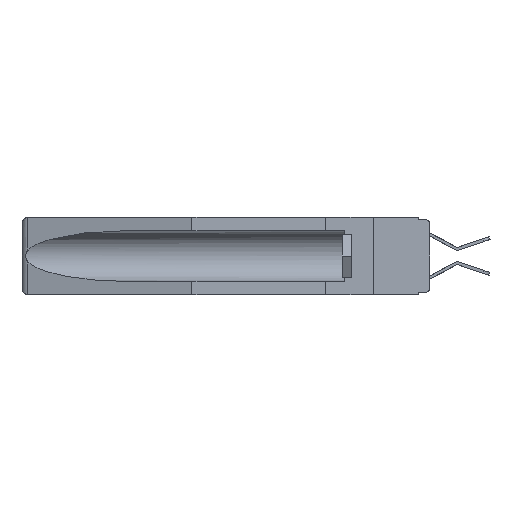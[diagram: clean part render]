
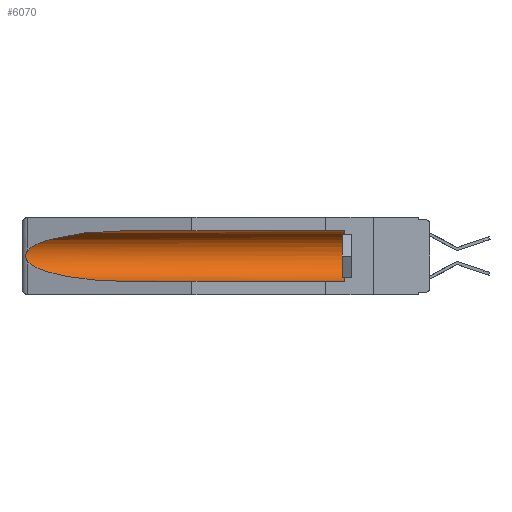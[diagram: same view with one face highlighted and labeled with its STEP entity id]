
A CAD part, left-side view. The second image highlights one B-rep face of the part: STEP entity #6070.
In plain terms, the highlighted cylindrical face has radius 2.857 mm (diameter 5.715 mm), a partial arc.
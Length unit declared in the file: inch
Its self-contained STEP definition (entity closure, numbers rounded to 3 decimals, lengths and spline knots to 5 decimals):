
#54 = EDGE_CURVE ( 'NONE', #11934, #7314, #14730, .T. ) ;
#150 = CARTESIAN_POINT ( 'NONE',  ( 0.21114, 1.30732, -0.059 ) ) ;
#220 =( BOUNDED_CURVE ( )  B_SPLINE_CURVE ( 3, ( #12397, #5140, #10967, #10677 ),
 .UNSPECIFIED., .F., .F. ) 
 B_SPLINE_CURVE_WITH_KNOTS ( ( 4, 4 ),
 ( 0.1948, 1.5708 ),
 .UNSPECIFIED. ) 
 CURVE ( )  GEOMETRIC_REPRESENTATION_ITEM ( )  RATIONAL_B_SPLINE_CURVE ( ( 1., 0.848, 0.848, 1. ) ) 
 REPRESENTATION_ITEM ( '' )  );
#445 = CARTESIAN_POINT ( 'NONE',  ( 0.2673, 1.5327, -0.16383 ) ) ;
#542 = ORIENTED_EDGE ( 'NONE', *, *, #2646, .T. ) ;
#723 = CARTESIAN_POINT ( 'NONE',  ( 0.2673, 1.53269, -0.17917 ) ) ;
#1757 = CARTESIAN_POINT ( 'NONE',  ( 0.155, 1.07973, -0.059 ) ) ;
#2565 = AXIS2_PLACEMENT_3D ( 'NONE', #5323, #18333, #18431 ) ;
#2646 = EDGE_CURVE ( 'NONE', #7314, #17627, #11357, .T. ) ;
#2702 = LINE ( 'NONE', #9964, #5491 ) ;
#3392 = DIRECTION ( 'NONE',  ( 0., 1., 0. ) ) ;
#3399 = CARTESIAN_POINT ( 'NONE',  ( 0.155, 0.126, -0.1715 ) ) ;
#4079 = AXIS2_PLACEMENT_3D ( 'NONE', #3399, #6447, #10950 ) ;
#4982 = ORIENTED_EDGE ( 'NONE', *, *, #9764, .T. ) ;
#5024 = CARTESIAN_POINT ( 'NONE',  ( 0.26597, 1.52961, -0.15275 ) ) ;
#5117 = CARTESIAN_POINT ( 'NONE',  ( 0.26537, 1.52718, -0.19328 ) ) ;
#5140 = CARTESIAN_POINT ( 'NONE',  ( 0.25451, 1.48313, -0.24835 ) ) ;
#5323 = CARTESIAN_POINT ( 'NONE',  ( 0.155, -0.30754, -0.1715 ) ) ;
#5491 = VECTOR ( 'NONE', #18487, 39.37008 ) ;
#6070 = ADVANCED_FACE ( 'NONE', ( #9517 ), #11938, .F. ) ;
#6447 = DIRECTION ( 'NONE',  ( 0., -1., 0. ) ) ;
#7170 = CARTESIAN_POINT ( 'NONE',  ( 0.155, 0.126, -0.284 ) ) ;
#7314 = VERTEX_POINT ( 'NONE', #8715 ) ;
#7609 = ORIENTED_EDGE ( 'NONE', *, *, #12559, .T. ) ;
#7975 = CARTESIAN_POINT ( 'NONE',  ( 0.26655, 1.53094, -0.18657 ) ) ;
#8081 = CARTESIAN_POINT ( 'NONE',  ( 0.2675, 1.53308, -0.17534 ) ) ;
#8715 = CARTESIAN_POINT ( 'NONE',  ( 0.26537, 1.52718, -0.14972 ) ) ;
#9391 = ORIENTED_EDGE ( 'NONE', *, *, #18700, .T. ) ;
#9517 = FACE_OUTER_BOUND ( 'NONE', #13673, .T. ) ;
#9764 = EDGE_CURVE ( 'NONE', #12864, #11934, #10479, .T. ) ;
#9964 = CARTESIAN_POINT ( 'NONE',  ( 0.155, -0.30754, -0.284 ) ) ;
#10094 = CARTESIAN_POINT ( 'NONE',  ( 0.25451, 1.48313, -0.09465 ) ) ;
#10386 = CARTESIAN_POINT ( 'NONE',  ( 0.155, 0.126, -0.059 ) ) ;
#10479 = LINE ( 'NONE', #15146, #15121 ) ;
#10677 = CARTESIAN_POINT ( 'NONE',  ( 0.155, 1.07973, -0.284 ) ) ;
#10950 = DIRECTION ( 'NONE',  ( 0., 0., 1. ) ) ;
#10967 = CARTESIAN_POINT ( 'NONE',  ( 0.21114, 1.30732, -0.284 ) ) ;
#11010 = CARTESIAN_POINT ( 'NONE',  ( 0.26537, 1.52718, -0.19328 ) ) ;
#11357 = B_SPLINE_CURVE_WITH_KNOTS ( 'NONE', 3,
 ( #16395, #5024, #17930, #445, #18025, #8081, #723, #7975, #15341, #5117 ),
 .UNSPECIFIED., .F., .F.,
 ( 4, 2, 2, 2, 4 ),
 ( 0., 0.00029, 0.00058, 0.00087, 0.00117 ),
 .UNSPECIFIED. ) ;
#11478 = ORIENTED_EDGE ( 'NONE', *, *, #54, .T. ) ;
#11934 = VERTEX_POINT ( 'NONE', #1757 ) ;
#11938 = CYLINDRICAL_SURFACE ( 'NONE', #2565, 0.1125 ) ;
#12397 = CARTESIAN_POINT ( 'NONE',  ( 0.26537, 1.52718, -0.19328 ) ) ;
#12559 = EDGE_CURVE ( 'NONE', #17627, #18204, #220, .T. ) ;
#12864 = VERTEX_POINT ( 'NONE', #10386 ) ;
#13048 = CARTESIAN_POINT ( 'NONE',  ( 0.26537, 1.52718, -0.14972 ) ) ;
#13358 = EDGE_CURVE ( 'NONE', #17990, #18204, #2702, .T. ) ;
#13450 = CARTESIAN_POINT ( 'NONE',  ( 0.155, 1.07973, -0.284 ) ) ;
#13673 = EDGE_LOOP ( 'NONE', ( #11478, #542, #7609, #14293, #9391, #4982 ) ) ;
#14293 = ORIENTED_EDGE ( 'NONE', *, *, #13358, .F. ) ;
#14730 =( BOUNDED_CURVE ( )  B_SPLINE_CURVE ( 3, ( #14770, #150, #10094, #13048 ),
 .UNSPECIFIED., .F., .F. ) 
 B_SPLINE_CURVE_WITH_KNOTS ( ( 4, 4 ),
 ( 4.71239, 6.08839 ),
 .UNSPECIFIED. ) 
 CURVE ( )  GEOMETRIC_REPRESENTATION_ITEM ( )  RATIONAL_B_SPLINE_CURVE ( ( 1., 0.848, 0.848, 1. ) ) 
 REPRESENTATION_ITEM ( '' )  );
#14770 = CARTESIAN_POINT ( 'NONE',  ( 0.155, 1.07973, -0.059 ) ) ;
#15121 = VECTOR ( 'NONE', #3392, 39.37008 ) ;
#15146 = CARTESIAN_POINT ( 'NONE',  ( 0.155, -0.30754, -0.059 ) ) ;
#15341 = CARTESIAN_POINT ( 'NONE',  ( 0.26597, 1.5296, -0.19026 ) ) ;
#15971 = CIRCLE ( 'NONE', #4079, 0.1125 ) ;
#16395 = CARTESIAN_POINT ( 'NONE',  ( 0.26537, 1.52718, -0.14972 ) ) ;
#17627 = VERTEX_POINT ( 'NONE', #11010 ) ;
#17930 = CARTESIAN_POINT ( 'NONE',  ( 0.26654, 1.53092, -0.15636 ) ) ;
#17990 = VERTEX_POINT ( 'NONE', #7170 ) ;
#18025 = CARTESIAN_POINT ( 'NONE',  ( 0.2675, 1.53308, -0.16763 ) ) ;
#18204 = VERTEX_POINT ( 'NONE', #13450 ) ;
#18333 = DIRECTION ( 'NONE',  ( 0., 1., 0. ) ) ;
#18431 = DIRECTION ( 'NONE',  ( 0., 0., 1. ) ) ;
#18487 = DIRECTION ( 'NONE',  ( 0., 1., 0. ) ) ;
#18700 = EDGE_CURVE ( 'NONE', #17990, #12864, #15971, .T. ) ;
